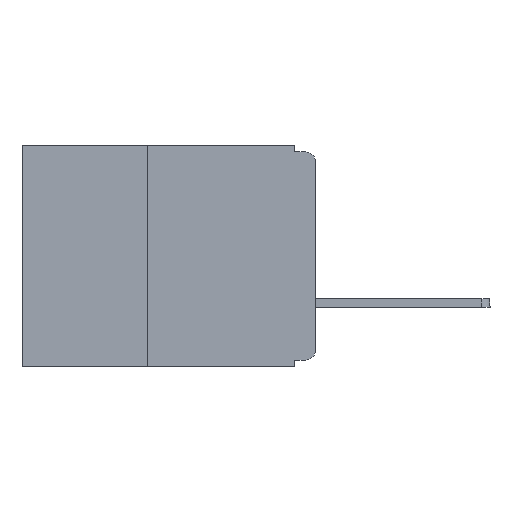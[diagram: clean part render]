
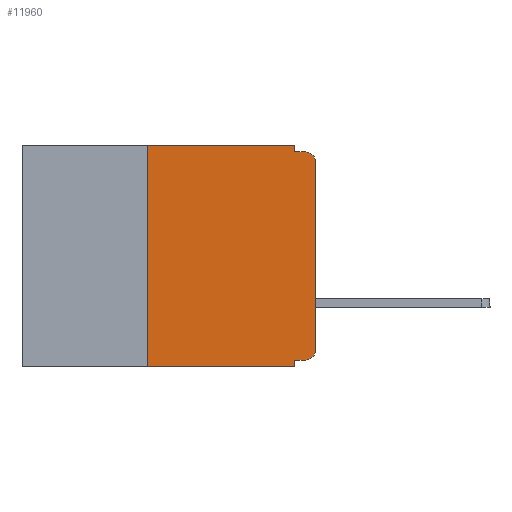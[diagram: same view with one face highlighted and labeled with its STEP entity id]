
A CAD part, left-side view. The second image highlights one B-rep face of the part: STEP entity #11960.
In plain terms, the highlighted planar face has unit normal (-1, 0, 0).
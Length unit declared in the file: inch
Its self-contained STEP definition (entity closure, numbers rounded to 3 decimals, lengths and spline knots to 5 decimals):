
#541 = CIRCLE ( 'NONE', #21024, 0.015 ) ;
#917 = CARTESIAN_POINT ( 'NONE',  ( 0., 0., -0.025 ) ) ;
#1126 = EDGE_CURVE ( 'NONE', #17097, #10975, #20610, .T. ) ;
#1979 = LINE ( 'NONE', #11563, #22579 ) ;
#2055 = VERTEX_POINT ( 'NONE', #4214 ) ;
#2358 = ORIENTED_EDGE ( 'NONE', *, *, #5803, .F. ) ;
#2752 = VERTEX_POINT ( 'NONE', #9201 ) ;
#2990 = DIRECTION ( 'NONE',  ( 0., 0., -1. ) ) ;
#2999 = LINE ( 'NONE', #11008, #18325 ) ;
#3241 = EDGE_CURVE ( 'NONE', #2752, #22729, #9900, .T. ) ;
#3451 = VERTEX_POINT ( 'NONE', #917 ) ;
#4214 = CARTESIAN_POINT ( 'NONE',  ( 0., 0.031, 0. ) ) ;
#4305 = VECTOR ( 'NONE', #7647, 39.37008 ) ;
#4360 = DIRECTION ( 'NONE',  ( 0., 0., 1. ) ) ;
#4478 = CARTESIAN_POINT ( 'NONE',  ( 0., 0., 0. ) ) ;
#4823 = ORIENTED_EDGE ( 'NONE', *, *, #19731, .F. ) ;
#4933 = EDGE_CURVE ( 'NONE', #9392, #3451, #7919, .T. ) ;
#4946 = VECTOR ( 'NONE', #20247, 39.37008 ) ;
#5119 = ORIENTED_EDGE ( 'NONE', *, *, #24018, .T. ) ;
#5803 = EDGE_CURVE ( 'NONE', #7687, #14111, #1979, .T. ) ;
#7292 = CIRCLE ( 'NONE', #20458, 0.015 ) ;
#7449 = CARTESIAN_POINT ( 'NONE',  ( 0., 0.031, -0.33 ) ) ;
#7647 = DIRECTION ( 'NONE',  ( 0., -1., 0. ) ) ;
#7687 = VERTEX_POINT ( 'NONE', #17408 ) ;
#7919 = LINE ( 'NONE', #4478, #12619 ) ;
#8109 = CARTESIAN_POINT ( 'NONE',  ( 0., 0., -0.01 ) ) ;
#8226 = DIRECTION ( 'NONE',  ( 0., -1., 0. ) ) ;
#8852 = DIRECTION ( 'NONE',  ( -1., 0., 0. ) ) ;
#9201 = CARTESIAN_POINT ( 'NONE',  ( 0., 0.031, -0.01 ) ) ;
#9203 = ORIENTED_EDGE ( 'NONE', *, *, #1126, .F. ) ;
#9223 = EDGE_CURVE ( 'NONE', #3451, #22729, #541, .T. ) ;
#9229 = DIRECTION ( 'NONE',  ( -1., 0., 0. ) ) ;
#9392 = VERTEX_POINT ( 'NONE', #15311 ) ;
#9849 = VECTOR ( 'NONE', #15195, 39.37008 ) ;
#9900 = LINE ( 'NONE', #8109, #13354 ) ;
#10817 = ORIENTED_EDGE ( 'NONE', *, *, #11777, .T. ) ;
#10975 = VERTEX_POINT ( 'NONE', #20821 ) ;
#11008 = CARTESIAN_POINT ( 'NONE',  ( 0., 0.031, -0.33 ) ) ;
#11178 = CARTESIAN_POINT ( 'NONE',  ( 0., 0.437, 0. ) ) ;
#11223 = DIRECTION ( 'NONE',  ( 0., 1., 0. ) ) ;
#11563 = CARTESIAN_POINT ( 'NONE',  ( 0., 0., -0.32 ) ) ;
#11777 = EDGE_CURVE ( 'NONE', #7687, #9392, #7292, .T. ) ;
#11830 = DIRECTION ( 'NONE',  ( 1., 0., 0. ) ) ;
#11907 = AXIS2_PLACEMENT_3D ( 'NONE', #23778, #11830, #25772 ) ;
#11960 = ADVANCED_FACE ( 'NONE', ( #13560 ), #19796, .F. ) ;
#12586 = ORIENTED_EDGE ( 'NONE', *, *, #4933, .T. ) ;
#12619 = VECTOR ( 'NONE', #4360, 39.37008 ) ;
#13354 = VECTOR ( 'NONE', #8226, 39.37008 ) ;
#13560 = FACE_OUTER_BOUND ( 'NONE', #14254, .T. ) ;
#14111 = VERTEX_POINT ( 'NONE', #19082 ) ;
#14137 = CARTESIAN_POINT ( 'NONE',  ( 0., 0.031, 0. ) ) ;
#14254 = EDGE_LOOP ( 'NONE', ( #12586, #20399, #19493, #17028, #22022, #9203, #5119, #4823, #2358, #10817 ) ) ;
#14619 = DIRECTION ( 'NONE',  ( 0., 0., 1. ) ) ;
#14679 = CARTESIAN_POINT ( 'NONE',  ( 0., 0.25, -0.33 ) ) ;
#15195 = DIRECTION ( 'NONE',  ( 0., -1., 0. ) ) ;
#15288 = VERTEX_POINT ( 'NONE', #7449 ) ;
#15311 = CARTESIAN_POINT ( 'NONE',  ( 0., 0., -0.305 ) ) ;
#16140 = EDGE_CURVE ( 'NONE', #2055, #2752, #20910, .T. ) ;
#17028 = ORIENTED_EDGE ( 'NONE', *, *, #16140, .F. ) ;
#17097 = VERTEX_POINT ( 'NONE', #21337 ) ;
#17206 = VECTOR ( 'NONE', #14619, 39.37008 ) ;
#17408 = CARTESIAN_POINT ( 'NONE',  ( 0., 0.015, -0.32 ) ) ;
#17727 = CARTESIAN_POINT ( 'NONE',  ( 0., 0.015, -0.01 ) ) ;
#18091 = EDGE_CURVE ( 'NONE', #10975, #2055, #25757, .T. ) ;
#18325 = VECTOR ( 'NONE', #2990, 39.37008 ) ;
#19082 = CARTESIAN_POINT ( 'NONE',  ( 0., 0.031, -0.32 ) ) ;
#19493 = ORIENTED_EDGE ( 'NONE', *, *, #3241, .F. ) ;
#19644 = LINE ( 'NONE', #21626, #4305 ) ;
#19731 = EDGE_CURVE ( 'NONE', #14111, #15288, #2999, .T. ) ;
#19796 = PLANE ( 'NONE',  #11907 ) ;
#20247 = DIRECTION ( 'NONE',  ( 0., 0., -1. ) ) ;
#20399 = ORIENTED_EDGE ( 'NONE', *, *, #9223, .T. ) ;
#20458 = AXIS2_PLACEMENT_3D ( 'NONE', #21199, #9229, #23192 ) ;
#20610 = LINE ( 'NONE', #14679, #17206 ) ;
#20819 = CARTESIAN_POINT ( 'NONE',  ( 0., 0.015, -0.025 ) ) ;
#20821 = CARTESIAN_POINT ( 'NONE',  ( 0., 0.25, 0. ) ) ;
#20910 = LINE ( 'NONE', #14137, #4946 ) ;
#21024 = AXIS2_PLACEMENT_3D ( 'NONE', #20819, #8852, #22825 ) ;
#21199 = CARTESIAN_POINT ( 'NONE',  ( 0., 0.015, -0.305 ) ) ;
#21337 = CARTESIAN_POINT ( 'NONE',  ( 0., 0.25, -0.33 ) ) ;
#21626 = CARTESIAN_POINT ( 'NONE',  ( 0., 0.437, -0.33 ) ) ;
#22022 = ORIENTED_EDGE ( 'NONE', *, *, #18091, .F. ) ;
#22579 = VECTOR ( 'NONE', #11223, 39.37008 ) ;
#22729 = VERTEX_POINT ( 'NONE', #17727 ) ;
#22825 = DIRECTION ( 'NONE',  ( 0., 0., -1. ) ) ;
#23192 = DIRECTION ( 'NONE',  ( 0., 0., -1. ) ) ;
#23778 = CARTESIAN_POINT ( 'NONE',  ( 0., 0.437, 0. ) ) ;
#24018 = EDGE_CURVE ( 'NONE', #17097, #15288, #19644, .T. ) ;
#25757 = LINE ( 'NONE', #11178, #9849 ) ;
#25772 = DIRECTION ( 'NONE',  ( 0., 0., -1. ) ) ;
